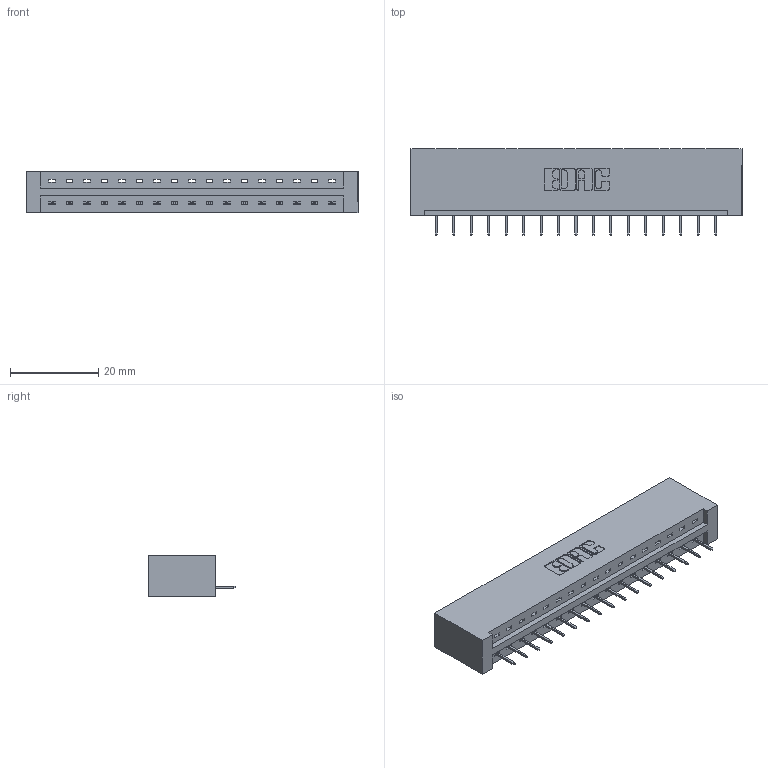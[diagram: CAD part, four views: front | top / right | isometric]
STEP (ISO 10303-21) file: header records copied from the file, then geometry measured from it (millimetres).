
FILE_DESCRIPTION (( 'STEP AP203' ), '1' );
FILE_NAME ('387-017-524-101.STEP', '2019-10-02T19:07:07', ( '' ), ( '' ), 'SwSTEP 2.0', 'SolidWorks 2016', '' );
FILE_SCHEMA (( 'CONFIG_CONTROL_DESIGN' ));
Length unit declared in the file: inch
Products named in the file (3): 337 Part_No Mounting Lugs; 387-017-524-101; 345-292-001_345-293-124
Assembly tree (18 placements, depth 2):
  387-017-524-101
    337 Part_No Mounting Lugs
    345-292-001_345-293-124  x17
Bounding box: 75.23 x 19.69 x 9.4 mm (x, y, z)
Volume: 8178.1 mm3; surface area: 8057.4 mm2
Topology: 18 solids, 18 shells, 1228 faces, 3551 edges, 2298 vertices
Faces by surface type: plane 950, cylinder 278
Entity records: 15667 total; most frequent: CARTESIAN_POINT 2733, ORIENTED_EDGE 2686, DIRECTION 2345, EDGE_CURVE 1343, LINE 1227, VECTOR 1227, VERTEX_POINT 890, AXIS2_PLACEMENT_3D 559
